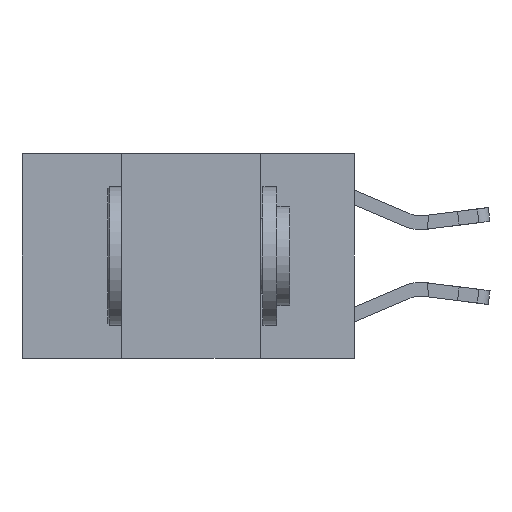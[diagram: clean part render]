
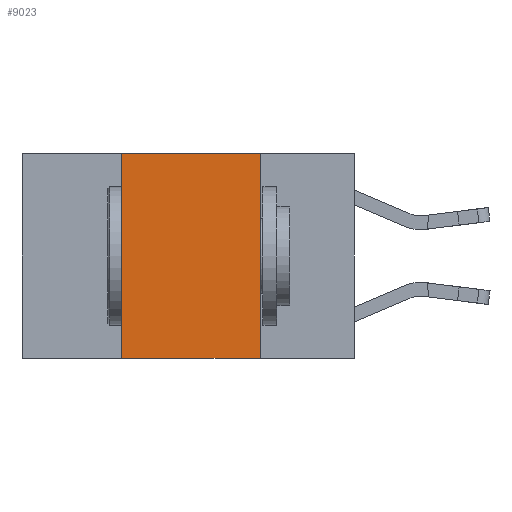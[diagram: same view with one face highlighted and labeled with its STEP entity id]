
A CAD part, left-side view. The second image highlights one B-rep face of the part: STEP entity #9023.
In plain terms, the highlighted planar face has unit normal (-1, 0, 0).
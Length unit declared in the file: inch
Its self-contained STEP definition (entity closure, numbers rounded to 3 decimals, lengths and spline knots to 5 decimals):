
#159 = ORIENTED_EDGE ( 'NONE', *, *, #10436, .T. ) ;
#1059 = EDGE_CURVE ( 'NONE', #3186, #1565, #1219, .T. ) ;
#1219 = LINE ( 'NONE', #9655, #12488 ) ;
#1565 = VERTEX_POINT ( 'NONE', #8820 ) ;
#1865 = DIRECTION ( 'NONE',  ( 1., 0., 0. ) ) ;
#1885 = VECTOR ( 'NONE', #9568, 39.37008 ) ;
#1908 = DIRECTION ( 'NONE',  ( 0., 0., -1. ) ) ;
#2352 = VECTOR ( 'NONE', #11831, 39.37008 ) ;
#2427 = CARTESIAN_POINT ( 'NONE',  ( 0., 0.42, 0. ) ) ;
#2973 = CARTESIAN_POINT ( 'NONE',  ( 0., 0.6, 0. ) ) ;
#3055 = CARTESIAN_POINT ( 'NONE',  ( 0., 0.6, -0.37 ) ) ;
#3181 = EDGE_LOOP ( 'NONE', ( #4343, #9477, #7092, #159 ) ) ;
#3186 = VERTEX_POINT ( 'NONE', #2427 ) ;
#3765 = DIRECTION ( 'NONE',  ( 0., -1., 0. ) ) ;
#4343 = ORIENTED_EDGE ( 'NONE', *, *, #10820, .F. ) ;
#5295 = CARTESIAN_POINT ( 'NONE',  ( 0., 0.42, 0. ) ) ;
#5660 = VECTOR ( 'NONE', #7975, 39.37008 ) ;
#6895 = CARTESIAN_POINT ( 'NONE',  ( 0., 0.17, 0. ) ) ;
#7092 = ORIENTED_EDGE ( 'NONE', *, *, #12607, .F. ) ;
#7376 = FACE_OUTER_BOUND ( 'NONE', #3181, .T. ) ;
#7790 = LINE ( 'NONE', #5295, #2352 ) ;
#7975 = DIRECTION ( 'NONE',  ( 0., 0., -1. ) ) ;
#8199 = VERTEX_POINT ( 'NONE', #10190 ) ;
#8634 = VERTEX_POINT ( 'NONE', #10952 ) ;
#8820 = CARTESIAN_POINT ( 'NONE',  ( 0., 0.17, 0. ) ) ;
#9023 = ADVANCED_FACE ( 'NONE', ( #7376 ), #13813, .F. ) ;
#9477 = ORIENTED_EDGE ( 'NONE', *, *, #1059, .F. ) ;
#9568 = DIRECTION ( 'NONE',  ( 0., -1., 0. ) ) ;
#9647 = AXIS2_PLACEMENT_3D ( 'NONE', #2973, #1865, #1908 ) ;
#9655 = CARTESIAN_POINT ( 'NONE',  ( 0., 0.6, 0. ) ) ;
#10190 = CARTESIAN_POINT ( 'NONE',  ( 0., 0.42, -0.37 ) ) ;
#10436 = EDGE_CURVE ( 'NONE', #8199, #8634, #13106, .T. ) ;
#10820 = EDGE_CURVE ( 'NONE', #1565, #8634, #11808, .T. ) ;
#10952 = CARTESIAN_POINT ( 'NONE',  ( 0., 0.17, -0.37 ) ) ;
#11808 = LINE ( 'NONE', #6895, #5660 ) ;
#11831 = DIRECTION ( 'NONE',  ( 0., 0., 1. ) ) ;
#12488 = VECTOR ( 'NONE', #3765, 39.37008 ) ;
#12607 = EDGE_CURVE ( 'NONE', #8199, #3186, #7790, .T. ) ;
#13106 = LINE ( 'NONE', #3055, #1885 ) ;
#13813 = PLANE ( 'NONE',  #9647 ) ;
